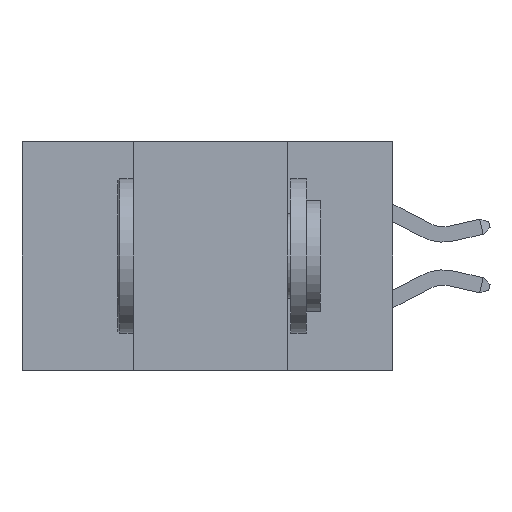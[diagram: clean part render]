
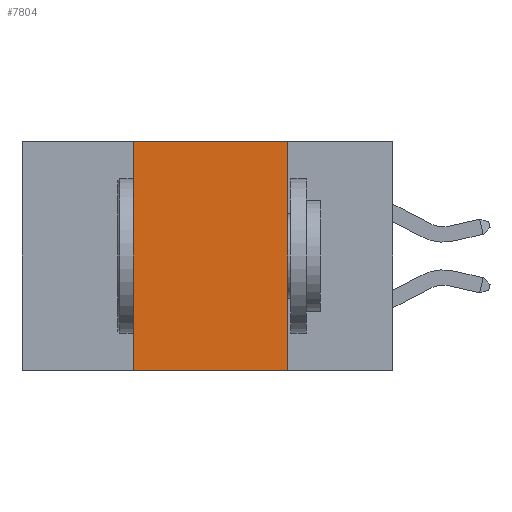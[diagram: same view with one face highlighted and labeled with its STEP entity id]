
A CAD part, left-side view. The second image highlights one B-rep face of the part: STEP entity #7804.
In plain terms, the highlighted planar face has unit normal (-1, 0, 0).
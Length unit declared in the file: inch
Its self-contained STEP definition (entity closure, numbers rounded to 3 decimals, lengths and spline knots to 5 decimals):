
#517 = DIRECTION ( 'NONE',  ( 0., -1., 0. ) ) ;
#2017 = CARTESIAN_POINT ( 'NONE',  ( 0., 0.17, 0. ) ) ;
#2230 = ORIENTED_EDGE ( 'NONE', *, *, #11692, .F. ) ;
#2431 = VERTEX_POINT ( 'NONE', #12279 ) ;
#2820 = CARTESIAN_POINT ( 'NONE',  ( 0., 0.42, 0. ) ) ;
#3158 = FACE_OUTER_BOUND ( 'NONE', #3369, .T. ) ;
#3369 = EDGE_LOOP ( 'NONE', ( #9009, #2230, #5867, #9438 ) ) ;
#4222 = DIRECTION ( 'NONE',  ( 0., 0., 1. ) ) ;
#4316 = VERTEX_POINT ( 'NONE', #7793 ) ;
#4618 = VECTOR ( 'NONE', #4222, 39.37008 ) ;
#5807 = VECTOR ( 'NONE', #15217, 39.37008 ) ;
#5867 = ORIENTED_EDGE ( 'NONE', *, *, #13244, .F. ) ;
#6140 = CARTESIAN_POINT ( 'NONE',  ( 0., 0.6, 0. ) ) ;
#6939 = DIRECTION ( 'NONE',  ( 1., 0., 0. ) ) ;
#7253 = LINE ( 'NONE', #7401, #9976 ) ;
#7401 = CARTESIAN_POINT ( 'NONE',  ( 0., 0.6, -0.37 ) ) ;
#7532 = DIRECTION ( 'NONE',  ( 0., 0., -1. ) ) ;
#7793 = CARTESIAN_POINT ( 'NONE',  ( 0., 0.42, 0. ) ) ;
#7804 = ADVANCED_FACE ( 'NONE', ( #3158 ), #10918, .F. ) ;
#8242 = CARTESIAN_POINT ( 'NONE',  ( 0., 0.6, 0. ) ) ;
#8320 = VERTEX_POINT ( 'NONE', #8736 ) ;
#8736 = CARTESIAN_POINT ( 'NONE',  ( 0., 0.17, -0.37 ) ) ;
#9009 = ORIENTED_EDGE ( 'NONE', *, *, #11718, .F. ) ;
#9018 = VERTEX_POINT ( 'NONE', #11362 ) ;
#9374 = LINE ( 'NONE', #6140, #5807 ) ;
#9392 = AXIS2_PLACEMENT_3D ( 'NONE', #8242, #6939, #15924 ) ;
#9438 = ORIENTED_EDGE ( 'NONE', *, *, #16271, .T. ) ;
#9976 = VECTOR ( 'NONE', #517, 39.37008 ) ;
#10904 = LINE ( 'NONE', #2820, #4618 ) ;
#10918 = PLANE ( 'NONE',  #9392 ) ;
#11362 = CARTESIAN_POINT ( 'NONE',  ( 0., 0.42, -0.37 ) ) ;
#11692 = EDGE_CURVE ( 'NONE', #4316, #2431, #9374, .T. ) ;
#11718 = EDGE_CURVE ( 'NONE', #2431, #8320, #15342, .T. ) ;
#12043 = VECTOR ( 'NONE', #7532, 39.37008 ) ;
#12279 = CARTESIAN_POINT ( 'NONE',  ( 0., 0.17, 0. ) ) ;
#13244 = EDGE_CURVE ( 'NONE', #9018, #4316, #10904, .T. ) ;
#15217 = DIRECTION ( 'NONE',  ( 0., -1., 0. ) ) ;
#15342 = LINE ( 'NONE', #2017, #12043 ) ;
#15924 = DIRECTION ( 'NONE',  ( 0., 0., -1. ) ) ;
#16271 = EDGE_CURVE ( 'NONE', #9018, #8320, #7253, .T. ) ;
